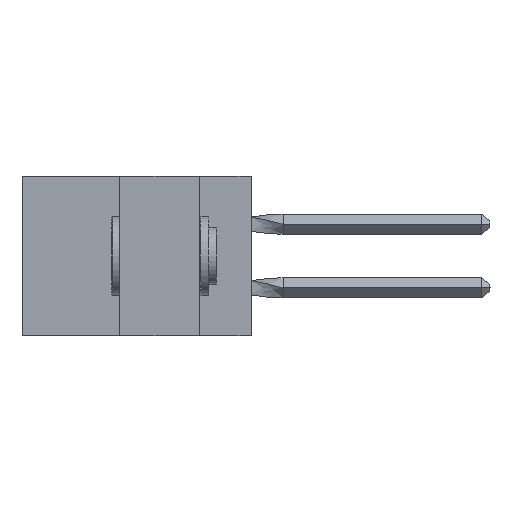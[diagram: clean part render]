
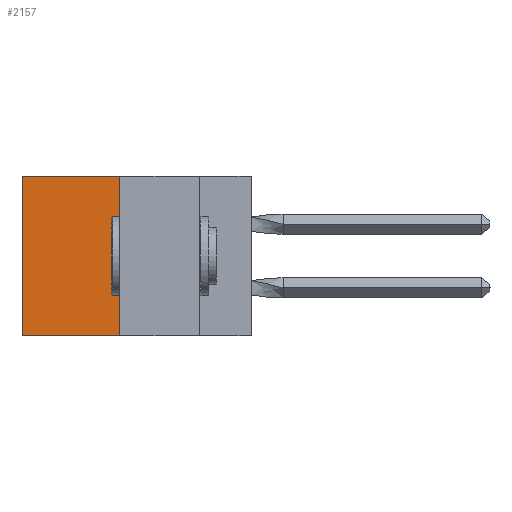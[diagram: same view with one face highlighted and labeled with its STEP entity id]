
A CAD part, left-side view. The second image highlights one B-rep face of the part: STEP entity #2157.
In plain terms, the highlighted planar face has unit normal (-1, 0, 0).
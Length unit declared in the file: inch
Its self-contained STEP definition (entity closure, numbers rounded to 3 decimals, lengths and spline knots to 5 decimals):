
#587 = PLANE ( 'NONE',  #7885 ) ;
#1853 = VERTEX_POINT ( 'NONE', #15612 ) ;
#2157 = ADVANCED_FACE ( 'NONE', ( #10872 ), #587, .F. ) ;
#3140 = CARTESIAN_POINT ( 'NONE',  ( 0.305, 0.413, 0. ) ) ;
#3449 = EDGE_CURVE ( 'NONE', #17791, #5720, #5462, .T. ) ;
#3712 = VERTEX_POINT ( 'NONE', #3140 ) ;
#5045 = ORIENTED_EDGE ( 'NONE', *, *, #6447, .F. ) ;
#5092 = CARTESIAN_POINT ( 'NONE',  ( 0.305, 0.413, -0.5 ) ) ;
#5462 = LINE ( 'NONE', #15629, #16716 ) ;
#5720 = VERTEX_POINT ( 'NONE', #12294 ) ;
#6447 = EDGE_CURVE ( 'NONE', #3712, #17791, #14192, .T. ) ;
#7454 = CARTESIAN_POINT ( 'NONE',  ( 0.305, 0.413, -0.5 ) ) ;
#7885 = AXIS2_PLACEMENT_3D ( 'NONE', #7454, #19375, #17561 ) ;
#8505 = LINE ( 'NONE', #18937, #13841 ) ;
#9840 = ORIENTED_EDGE ( 'NONE', *, *, #19544, .T. ) ;
#9885 = CARTESIAN_POINT ( 'NONE',  ( 0.305, 0.413, 0. ) ) ;
#10872 = FACE_OUTER_BOUND ( 'NONE', #11237, .T. ) ;
#11237 = EDGE_LOOP ( 'NONE', ( #22057, #15033, #5045, #9840 ) ) ;
#11869 = DIRECTION ( 'NONE',  ( 0., 0., -1. ) ) ;
#12294 = CARTESIAN_POINT ( 'NONE',  ( 0.305, 0.72, -0.5 ) ) ;
#13174 = DIRECTION ( 'NONE',  ( 0., 1., 0. ) ) ;
#13323 = LINE ( 'NONE', #9885, #21368 ) ;
#13841 = VECTOR ( 'NONE', #22070, 39.37008 ) ;
#14192 = LINE ( 'NONE', #5092, #17429 ) ;
#14672 = EDGE_CURVE ( 'NONE', #1853, #5720, #8505, .T. ) ;
#15033 = ORIENTED_EDGE ( 'NONE', *, *, #3449, .F. ) ;
#15612 = CARTESIAN_POINT ( 'NONE',  ( 0.305, 0.72, 0. ) ) ;
#15629 = CARTESIAN_POINT ( 'NONE',  ( 0.305, 0.413, -0.5 ) ) ;
#16716 = VECTOR ( 'NONE', #19116, 39.37008 ) ;
#17429 = VECTOR ( 'NONE', #11869, 39.37008 ) ;
#17561 = DIRECTION ( 'NONE',  ( 0., 0., -1. ) ) ;
#17791 = VERTEX_POINT ( 'NONE', #18784 ) ;
#18784 = CARTESIAN_POINT ( 'NONE',  ( 0.305, 0.413, -0.5 ) ) ;
#18937 = CARTESIAN_POINT ( 'NONE',  ( 0.305, 0.72, -0.5 ) ) ;
#19116 = DIRECTION ( 'NONE',  ( 0., 1., 0. ) ) ;
#19375 = DIRECTION ( 'NONE',  ( 1., 0., 0. ) ) ;
#19544 = EDGE_CURVE ( 'NONE', #3712, #1853, #13323, .T. ) ;
#21368 = VECTOR ( 'NONE', #13174, 39.37008 ) ;
#22057 = ORIENTED_EDGE ( 'NONE', *, *, #14672, .T. ) ;
#22070 = DIRECTION ( 'NONE',  ( 0., 0., -1. ) ) ;
